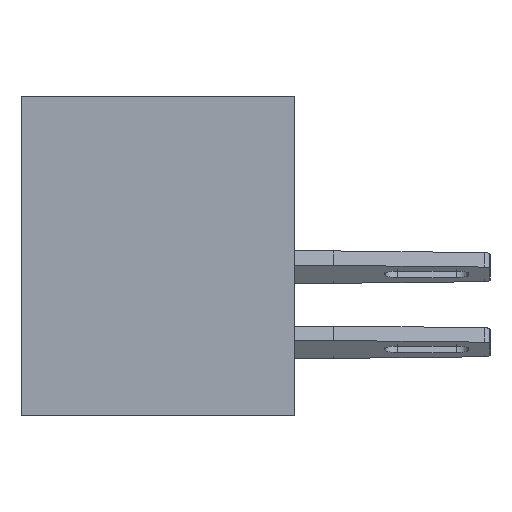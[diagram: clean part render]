
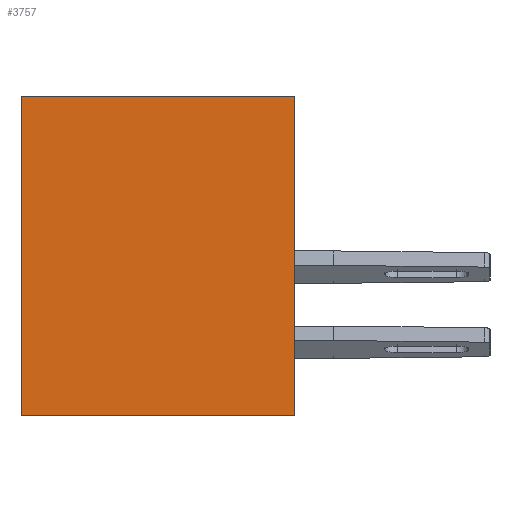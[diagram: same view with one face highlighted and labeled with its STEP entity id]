
A CAD part, left-side view. The second image highlights one B-rep face of the part: STEP entity #3757.
In plain terms, the highlighted planar face has unit normal (-1, 0, 0).
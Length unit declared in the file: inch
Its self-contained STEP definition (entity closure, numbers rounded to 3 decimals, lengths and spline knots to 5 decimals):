
#633 = VECTOR ( 'NONE', #22920, 39.37008 ) ;
#2378 = CARTESIAN_POINT ( 'NONE',  ( 0., 0., 0. ) ) ;
#2380 = LINE ( 'NONE', #20769, #20788 ) ;
#2384 = CARTESIAN_POINT ( 'NONE',  ( 0., 0., -0.531 ) ) ;
#2655 = EDGE_CURVE ( 'NONE', #6107, #10576, #12244, .T. ) ;
#3252 = VERTEX_POINT ( 'NONE', #7302 ) ;
#3757 = ADVANCED_FACE ( 'NONE', ( #20002 ), #19276, .F. ) ;
#4021 = EDGE_CURVE ( 'NONE', #3252, #10313, #19416, .T. ) ;
#6107 = VERTEX_POINT ( 'NONE', #16552 ) ;
#7185 = VECTOR ( 'NONE', #9432, 39.37008 ) ;
#7302 = CARTESIAN_POINT ( 'NONE',  ( 0., 0.453, 0. ) ) ;
#8278 = EDGE_CURVE ( 'NONE', #6107, #3252, #12071, .T. ) ;
#9432 = DIRECTION ( 'NONE',  ( 0., -1., 0. ) ) ;
#10313 = VERTEX_POINT ( 'NONE', #2378 ) ;
#10428 = ORIENTED_EDGE ( 'NONE', *, *, #4021, .F. ) ;
#10576 = VERTEX_POINT ( 'NONE', #2384 ) ;
#10870 = VECTOR ( 'NONE', #20323, 39.37008 ) ;
#11447 = CARTESIAN_POINT ( 'NONE',  ( 0., 0.453, -0.531 ) ) ;
#11995 = EDGE_CURVE ( 'NONE', #10576, #10313, #2380, .T. ) ;
#12071 = LINE ( 'NONE', #13909, #633 ) ;
#12244 = LINE ( 'NONE', #11447, #10870 ) ;
#12255 = DIRECTION ( 'NONE',  ( 0., 0., -1. ) ) ;
#13592 = DIRECTION ( 'NONE',  ( 0., 0., 1. ) ) ;
#13909 = CARTESIAN_POINT ( 'NONE',  ( 0., 0.453, 0. ) ) ;
#15695 = DIRECTION ( 'NONE',  ( 1., 0., 0. ) ) ;
#16519 = CARTESIAN_POINT ( 'NONE',  ( 0., 0.453, 0. ) ) ;
#16552 = CARTESIAN_POINT ( 'NONE',  ( 0., 0.453, -0.531 ) ) ;
#18705 = EDGE_LOOP ( 'NONE', ( #19192, #10428, #21988, #19655 ) ) ;
#19026 = AXIS2_PLACEMENT_3D ( 'NONE', #22915, #15695, #12255 ) ;
#19192 = ORIENTED_EDGE ( 'NONE', *, *, #11995, .T. ) ;
#19276 = PLANE ( 'NONE',  #19026 ) ;
#19416 = LINE ( 'NONE', #16519, #7185 ) ;
#19655 = ORIENTED_EDGE ( 'NONE', *, *, #2655, .T. ) ;
#20002 = FACE_OUTER_BOUND ( 'NONE', #18705, .T. ) ;
#20323 = DIRECTION ( 'NONE',  ( 0., -1., 0. ) ) ;
#20769 = CARTESIAN_POINT ( 'NONE',  ( 0., 0., 0. ) ) ;
#20788 = VECTOR ( 'NONE', #13592, 39.37008 ) ;
#21988 = ORIENTED_EDGE ( 'NONE', *, *, #8278, .F. ) ;
#22915 = CARTESIAN_POINT ( 'NONE',  ( 0., 0.453, 0. ) ) ;
#22920 = DIRECTION ( 'NONE',  ( 0., 0., 1. ) ) ;
